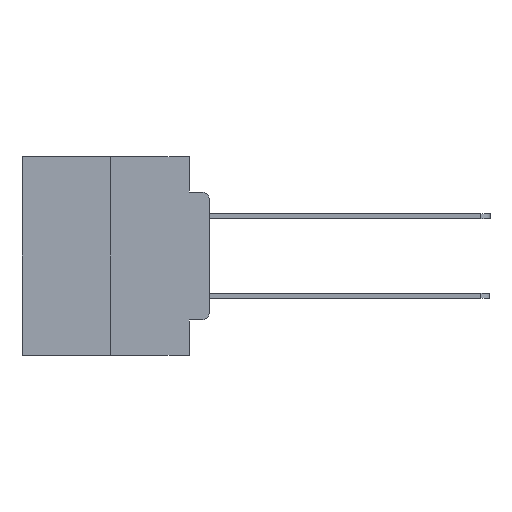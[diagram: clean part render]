
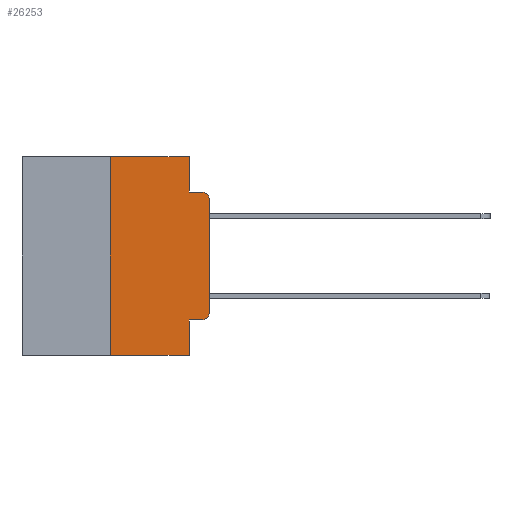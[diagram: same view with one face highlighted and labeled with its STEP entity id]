
A CAD part, left-side view. The second image highlights one B-rep face of the part: STEP entity #26253.
In plain terms, the highlighted planar face has unit normal (-1, 0, 0).
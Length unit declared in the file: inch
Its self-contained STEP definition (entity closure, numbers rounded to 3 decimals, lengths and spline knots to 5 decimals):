
#92 = DIRECTION ( 'NONE',  ( 0., 0., -1. ) ) ;
#145 = VERTEX_POINT ( 'NONE', #23993 ) ;
#260 = EDGE_CURVE ( 'NONE', #13930, #145, #561, .T. ) ;
#561 = LINE ( 'NONE', #12169, #21416 ) ;
#1357 = VERTEX_POINT ( 'NONE', #27049 ) ;
#2527 = ORIENTED_EDGE ( 'NONE', *, *, #25593, .F. ) ;
#3343 = DIRECTION ( 'NONE',  ( -1., 0., 0. ) ) ;
#3372 = EDGE_CURVE ( 'NONE', #13930, #21795, #27591, .T. ) ;
#3969 = VECTOR ( 'NONE', #92, 39.37008 ) ;
#4896 = EDGE_CURVE ( 'NONE', #21795, #14729, #14163, .T. ) ;
#4954 = VECTOR ( 'NONE', #9279, 39.37008 ) ;
#5391 = ORIENTED_EDGE ( 'NONE', *, *, #13775, .T. ) ;
#5557 = CARTESIAN_POINT ( 'NONE',  ( 0., 0.25, 0. ) ) ;
#6338 = LINE ( 'NONE', #17775, #4954 ) ;
#6495 = AXIS2_PLACEMENT_3D ( 'NONE', #22750, #9936, #24901 ) ;
#7099 = CIRCLE ( 'NONE', #17110, 0.02 ) ;
#7230 = CARTESIAN_POINT ( 'NONE',  ( 0., 0., 0. ) ) ;
#8125 = VERTEX_POINT ( 'NONE', #21538 ) ;
#8206 = EDGE_CURVE ( 'NONE', #8125, #10520, #26802, .T. ) ;
#8452 = AXIS2_PLACEMENT_3D ( 'NONE', #24076, #26224, #13443 ) ;
#8785 = VERTEX_POINT ( 'NONE', #17364 ) ;
#9279 = DIRECTION ( 'NONE',  ( 0., -1., 0. ) ) ;
#9761 = CARTESIAN_POINT ( 'NONE',  ( 0., 0.051, -0.4115 ) ) ;
#9936 = DIRECTION ( 'NONE',  ( -1., 0., 0. ) ) ;
#10520 = VERTEX_POINT ( 'NONE', #27823 ) ;
#12019 = DIRECTION ( 'NONE',  ( 0., 0., 1. ) ) ;
#12169 = CARTESIAN_POINT ( 'NONE',  ( 0., 0.051, 0. ) ) ;
#12784 = VECTOR ( 'NONE', #28149, 39.37008 ) ;
#12795 = CARTESIAN_POINT ( 'NONE',  ( 0., 0., -0.3915 ) ) ;
#13443 = DIRECTION ( 'NONE',  ( 0., 0., -1. ) ) ;
#13485 = CARTESIAN_POINT ( 'NONE',  ( 0., 0., -0.1085 ) ) ;
#13775 = EDGE_CURVE ( 'NONE', #1357, #145, #6338, .T. ) ;
#13930 = VERTEX_POINT ( 'NONE', #14033 ) ;
#14033 = CARTESIAN_POINT ( 'NONE',  ( 0., 0.051, -0.4115 ) ) ;
#14163 = CIRCLE ( 'NONE', #6495, 0.02 ) ;
#14729 = VERTEX_POINT ( 'NONE', #12795 ) ;
#15249 = CARTESIAN_POINT ( 'NONE',  ( 0., 0.051, -0.0885 ) ) ;
#15538 = ORIENTED_EDGE ( 'NONE', *, *, #8206, .F. ) ;
#16341 = VERTEX_POINT ( 'NONE', #15249 ) ;
#16371 = CARTESIAN_POINT ( 'NONE',  ( 0., 0.02, -0.1085 ) ) ;
#16431 = LINE ( 'NONE', #17607, #21468 ) ;
#17010 = EDGE_CURVE ( 'NONE', #14729, #27462, #21966, .T. ) ;
#17110 = AXIS2_PLACEMENT_3D ( 'NONE', #16371, #3343, #18511 ) ;
#17364 = CARTESIAN_POINT ( 'NONE',  ( 0., 0.02, -0.0885 ) ) ;
#17527 = ORIENTED_EDGE ( 'NONE', *, *, #260, .F. ) ;
#17607 = CARTESIAN_POINT ( 'NONE',  ( 0., 0.051, -0.0885 ) ) ;
#17775 = CARTESIAN_POINT ( 'NONE',  ( 0., 0.473, -0.5 ) ) ;
#18437 = VECTOR ( 'NONE', #12019, 39.37008 ) ;
#18446 = EDGE_CURVE ( 'NONE', #27462, #8785, #7099, .T. ) ;
#18511 = DIRECTION ( 'NONE',  ( 0., 0., -1. ) ) ;
#18523 = ORIENTED_EDGE ( 'NONE', *, *, #21337, .F. ) ;
#18861 = ORIENTED_EDGE ( 'NONE', *, *, #4896, .T. ) ;
#19100 = LINE ( 'NONE', #5557, #18437 ) ;
#19758 = DIRECTION ( 'NONE',  ( 0., -1., 0. ) ) ;
#21132 = EDGE_LOOP ( 'NONE', ( #27192, #23518, #18523, #2527, #15538, #21230, #5391, #17527, #23863, #18861 ) ) ;
#21226 = LINE ( 'NONE', #26163, #3969 ) ;
#21230 = ORIENTED_EDGE ( 'NONE', *, *, #27023, .F. ) ;
#21337 = EDGE_CURVE ( 'NONE', #16341, #8785, #16431, .T. ) ;
#21416 = VECTOR ( 'NONE', #27210, 39.37008 ) ;
#21468 = VECTOR ( 'NONE', #19758, 39.37008 ) ;
#21513 = FACE_OUTER_BOUND ( 'NONE', #21132, .T. ) ;
#21538 = CARTESIAN_POINT ( 'NONE',  ( 0., 0.25, 0. ) ) ;
#21723 = CARTESIAN_POINT ( 'NONE',  ( 0., 0.02, -0.4115 ) ) ;
#21795 = VERTEX_POINT ( 'NONE', #21723 ) ;
#21812 = CARTESIAN_POINT ( 'NONE',  ( 0., 0.473, 0. ) ) ;
#21954 = PLANE ( 'NONE',  #8452 ) ;
#21966 = LINE ( 'NONE', #7230, #26949 ) ;
#22588 = DIRECTION ( 'NONE',  ( 0., -1., 0. ) ) ;
#22750 = CARTESIAN_POINT ( 'NONE',  ( 0., 0.02, -0.3915 ) ) ;
#23518 = ORIENTED_EDGE ( 'NONE', *, *, #18446, .T. ) ;
#23863 = ORIENTED_EDGE ( 'NONE', *, *, #3372, .T. ) ;
#23993 = CARTESIAN_POINT ( 'NONE',  ( 0., 0.051, -0.5 ) ) ;
#24076 = CARTESIAN_POINT ( 'NONE',  ( 0., 0.473, 0. ) ) ;
#24377 = DIRECTION ( 'NONE',  ( 0., 0., 1. ) ) ;
#24901 = DIRECTION ( 'NONE',  ( 0., 0., -1. ) ) ;
#25593 = EDGE_CURVE ( 'NONE', #10520, #16341, #21226, .T. ) ;
#26163 = CARTESIAN_POINT ( 'NONE',  ( 0., 0.051, 0. ) ) ;
#26224 = DIRECTION ( 'NONE',  ( 1., 0., 0. ) ) ;
#26253 = ADVANCED_FACE ( 'NONE', ( #21513 ), #21954, .F. ) ;
#26802 = LINE ( 'NONE', #21812, #12784 ) ;
#26930 = VECTOR ( 'NONE', #22588, 39.37008 ) ;
#26949 = VECTOR ( 'NONE', #24377, 39.37008 ) ;
#27023 = EDGE_CURVE ( 'NONE', #1357, #8125, #19100, .T. ) ;
#27049 = CARTESIAN_POINT ( 'NONE',  ( 0., 0.25, -0.5 ) ) ;
#27192 = ORIENTED_EDGE ( 'NONE', *, *, #17010, .T. ) ;
#27210 = DIRECTION ( 'NONE',  ( 0., 0., -1. ) ) ;
#27462 = VERTEX_POINT ( 'NONE', #13485 ) ;
#27591 = LINE ( 'NONE', #9761, #26930 ) ;
#27823 = CARTESIAN_POINT ( 'NONE',  ( 0., 0.051, 0. ) ) ;
#28149 = DIRECTION ( 'NONE',  ( 0., -1., 0. ) ) ;
